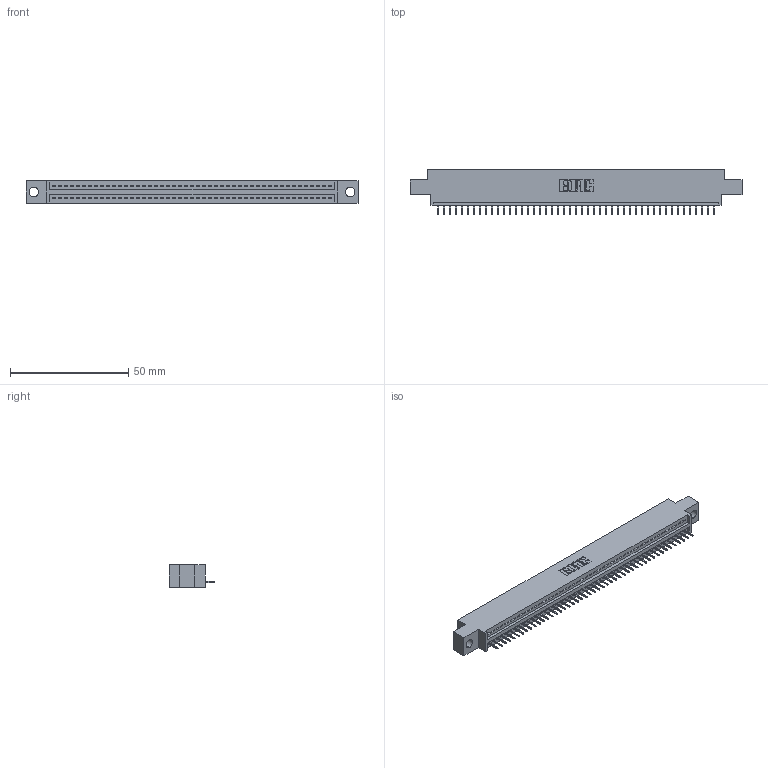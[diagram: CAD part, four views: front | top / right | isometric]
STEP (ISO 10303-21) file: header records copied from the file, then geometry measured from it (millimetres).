
FILE_DESCRIPTION (( 'STEP AP203' ), '1' );
FILE_NAME ('395-047-524-604.STEP', '2021-05-31T15:15:02', ( '' ), ( '' ), 'SwSTEP 2.0', 'SolidWorks 2020', '' );
FILE_SCHEMA (( 'CONFIG_CONTROL_DESIGN' ));
Length unit declared in the file: inch
Products named in the file (3): 395-047-524-604; 345 Part_0.170 Offset - 0.156 Dia-TI; 345-292-001_345-293-124
Assembly tree (48 placements, depth 2):
  395-047-524-604
    345 Part_0.170 Offset - 0.156 Dia-TI
    345-292-001_345-293-124  x47
Bounding box: 140.59 x 19.35 x 9.4 mm (x, y, z)
Volume: 12989.3 mm3; surface area: 16704.9 mm2
Topology: 48 solids, 48 shells, 3058 faces, 8849 edges, 5710 vertices
Faces by surface type: plane 2260, cylinder 798
Entity records: 35325 total; most frequent: CARTESIAN_POINT 6127, ORIENTED_EDGE 6106, DIRECTION 5343, EDGE_CURVE 3053, LINE 2737, VECTOR 2737, VERTEX_POINT 2030, AXIS2_PLACEMENT_3D 1303
